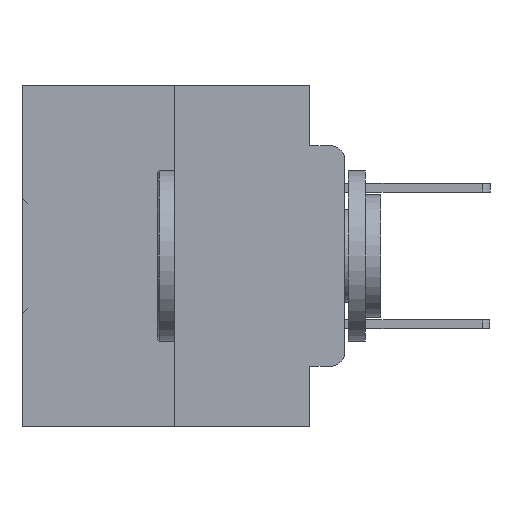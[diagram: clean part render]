
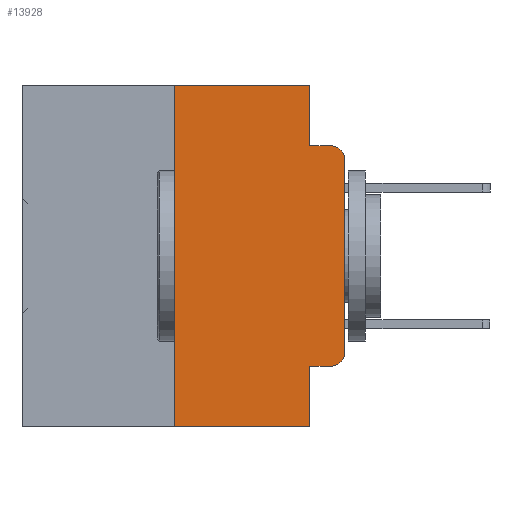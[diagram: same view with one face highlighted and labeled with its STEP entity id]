
A CAD part, left-side view. The second image highlights one B-rep face of the part: STEP entity #13928.
In plain terms, the highlighted planar face has unit normal (-1, 0, 0).
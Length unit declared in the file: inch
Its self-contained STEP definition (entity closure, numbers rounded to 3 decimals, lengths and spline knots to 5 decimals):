
#416 = ORIENTED_EDGE ( 'NONE', *, *, #15637, .F. ) ;
#2224 = VECTOR ( 'NONE', #7756, 39.37008 ) ;
#2241 = AXIS2_PLACEMENT_3D ( 'NONE', #5709, #25200, #8542 ) ;
#2367 = LINE ( 'NONE', #8130, #15496 ) ;
#3314 = LINE ( 'NONE', #32796, #31183 ) ;
#3437 = CARTESIAN_POINT ( 'NONE',  ( 0., 0.051, 0. ) ) ;
#5279 = VECTOR ( 'NONE', #13563, 39.37008 ) ;
#5709 = CARTESIAN_POINT ( 'NONE',  ( 0., 0.02, -0.1085 ) ) ;
#5865 = ORIENTED_EDGE ( 'NONE', *, *, #19171, .F. ) ;
#6052 = EDGE_CURVE ( 'NONE', #30944, #22599, #32962, .T. ) ;
#6305 = CARTESIAN_POINT ( 'NONE',  ( 0., 0.051, 0. ) ) ;
#7756 = DIRECTION ( 'NONE',  ( 0., -1., 0. ) ) ;
#8130 = CARTESIAN_POINT ( 'NONE',  ( 0., 0.051, 0. ) ) ;
#8542 = DIRECTION ( 'NONE',  ( 0., 0., -1. ) ) ;
#8615 = CARTESIAN_POINT ( 'NONE',  ( 0., 0.02, -0.0885 ) ) ;
#8648 = ORIENTED_EDGE ( 'NONE', *, *, #21038, .F. ) ;
#8674 = CARTESIAN_POINT ( 'NONE',  ( 0., 0.02, -0.3915 ) ) ;
#8835 = ORIENTED_EDGE ( 'NONE', *, *, #6052, .T. ) ;
#8892 = DIRECTION ( 'NONE',  ( 0., 0., -1. ) ) ;
#9800 = EDGE_CURVE ( 'NONE', #23290, #30944, #33865, .T. ) ;
#10785 = CARTESIAN_POINT ( 'NONE',  ( 0., 0.473, -0.5 ) ) ;
#11238 = CARTESIAN_POINT ( 'NONE',  ( 0., 0.473, 0. ) ) ;
#11444 = DIRECTION ( 'NONE',  ( 0., 0., -1. ) ) ;
#11486 = CARTESIAN_POINT ( 'NONE',  ( 0., 0., -0.1085 ) ) ;
#11658 = EDGE_CURVE ( 'NONE', #23290, #28032, #32495, .T. ) ;
#11702 = CARTESIAN_POINT ( 'NONE',  ( 0., 0.25, 0. ) ) ;
#11770 = ORIENTED_EDGE ( 'NONE', *, *, #28432, .T. ) ;
#11840 = ORIENTED_EDGE ( 'NONE', *, *, #26591, .T. ) ;
#12005 = DIRECTION ( 'NONE',  ( 0., 0., -1. ) ) ;
#12150 = AXIS2_PLACEMENT_3D ( 'NONE', #8674, #28113, #11444 ) ;
#12309 = ORIENTED_EDGE ( 'NONE', *, *, #9800, .T. ) ;
#12962 = CARTESIAN_POINT ( 'NONE',  ( 0., 0.051, -0.4115 ) ) ;
#13563 = DIRECTION ( 'NONE',  ( 0., -1., 0. ) ) ;
#13928 = ADVANCED_FACE ( 'NONE', ( #15236 ), #14042, .F. ) ;
#14042 = PLANE ( 'NONE',  #28378 ) ;
#15236 = FACE_OUTER_BOUND ( 'NONE', #26536, .T. ) ;
#15496 = VECTOR ( 'NONE', #30322, 39.37008 ) ;
#15637 = EDGE_CURVE ( 'NONE', #19413, #21071, #18611, .T. ) ;
#16198 = CARTESIAN_POINT ( 'NONE',  ( 0., 0.473, 0. ) ) ;
#16856 = DIRECTION ( 'NONE',  ( 1., 0., 0. ) ) ;
#17260 = EDGE_CURVE ( 'NONE', #29937, #19413, #31896, .T. ) ;
#18611 = LINE ( 'NONE', #16198, #32436 ) ;
#19036 = DIRECTION ( 'NONE',  ( 0., -1., 0. ) ) ;
#19171 = EDGE_CURVE ( 'NONE', #21071, #21282, #2367, .T. ) ;
#19413 = VERTEX_POINT ( 'NONE', #28639 ) ;
#21038 = EDGE_CURVE ( 'NONE', #21282, #21667, #35685, .T. ) ;
#21047 = LINE ( 'NONE', #10785, #5279 ) ;
#21071 = VERTEX_POINT ( 'NONE', #6305 ) ;
#21277 = VERTEX_POINT ( 'NONE', #11486 ) ;
#21282 = VERTEX_POINT ( 'NONE', #28162 ) ;
#21522 = EDGE_CURVE ( 'NONE', #29937, #28032, #21047, .T. ) ;
#21667 = VERTEX_POINT ( 'NONE', #8615 ) ;
#21717 = ORIENTED_EDGE ( 'NONE', *, *, #11658, .F. ) ;
#22599 = VERTEX_POINT ( 'NONE', #29572 ) ;
#22851 = CARTESIAN_POINT ( 'NONE',  ( 0., 0.051, -0.5 ) ) ;
#22989 = CARTESIAN_POINT ( 'NONE',  ( 0., 0.051, -0.4115 ) ) ;
#23290 = VERTEX_POINT ( 'NONE', #12962 ) ;
#24434 = CARTESIAN_POINT ( 'NONE',  ( 0., 0.051, -0.0885 ) ) ;
#25183 = VECTOR ( 'NONE', #12005, 39.37008 ) ;
#25200 = DIRECTION ( 'NONE',  ( -1., 0., 0. ) ) ;
#25696 = VECTOR ( 'NONE', #31289, 39.37008 ) ;
#26536 = EDGE_LOOP ( 'NONE', ( #11770, #11840, #8648, #5865, #416, #27541, #26576, #21717, #12309, #8835 ) ) ;
#26576 = ORIENTED_EDGE ( 'NONE', *, *, #21522, .T. ) ;
#26591 = EDGE_CURVE ( 'NONE', #21277, #21667, #33893, .T. ) ;
#27541 = ORIENTED_EDGE ( 'NONE', *, *, #17260, .F. ) ;
#28032 = VERTEX_POINT ( 'NONE', #22851 ) ;
#28113 = DIRECTION ( 'NONE',  ( -1., 0., 0. ) ) ;
#28162 = CARTESIAN_POINT ( 'NONE',  ( 0., 0.051, -0.0885 ) ) ;
#28378 = AXIS2_PLACEMENT_3D ( 'NONE', #11238, #16856, #8892 ) ;
#28432 = EDGE_CURVE ( 'NONE', #22599, #21277, #3314, .T. ) ;
#28639 = CARTESIAN_POINT ( 'NONE',  ( 0., 0.25, 0. ) ) ;
#28756 = CARTESIAN_POINT ( 'NONE',  ( 0., 0.25, -0.5 ) ) ;
#29572 = CARTESIAN_POINT ( 'NONE',  ( 0., 0., -0.3915 ) ) ;
#29937 = VERTEX_POINT ( 'NONE', #28756 ) ;
#30322 = DIRECTION ( 'NONE',  ( 0., 0., -1. ) ) ;
#30944 = VERTEX_POINT ( 'NONE', #35671 ) ;
#31037 = VECTOR ( 'NONE', #33870, 39.37008 ) ;
#31183 = VECTOR ( 'NONE', #35534, 39.37008 ) ;
#31289 = DIRECTION ( 'NONE',  ( 0., -1., 0. ) ) ;
#31896 = LINE ( 'NONE', #11702, #31037 ) ;
#32436 = VECTOR ( 'NONE', #19036, 39.37008 ) ;
#32495 = LINE ( 'NONE', #3437, #25183 ) ;
#32796 = CARTESIAN_POINT ( 'NONE',  ( 0., 0., 0. ) ) ;
#32962 = CIRCLE ( 'NONE', #12150, 0.02 ) ;
#33865 = LINE ( 'NONE', #22989, #25696 ) ;
#33870 = DIRECTION ( 'NONE',  ( 0., 0., 1. ) ) ;
#33893 = CIRCLE ( 'NONE', #2241, 0.02 ) ;
#35534 = DIRECTION ( 'NONE',  ( 0., 0., 1. ) ) ;
#35671 = CARTESIAN_POINT ( 'NONE',  ( 0., 0.02, -0.4115 ) ) ;
#35685 = LINE ( 'NONE', #24434, #2224 ) ;
